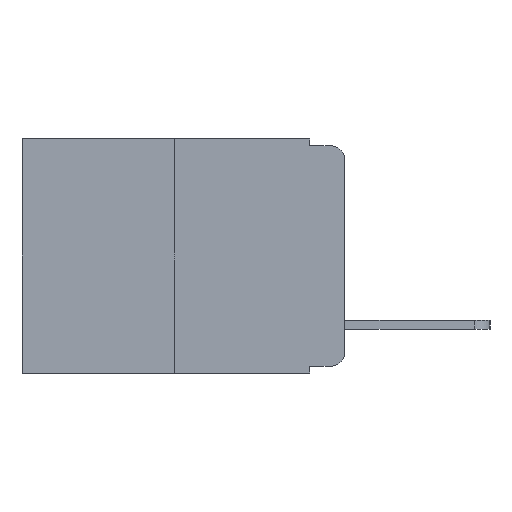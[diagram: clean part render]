
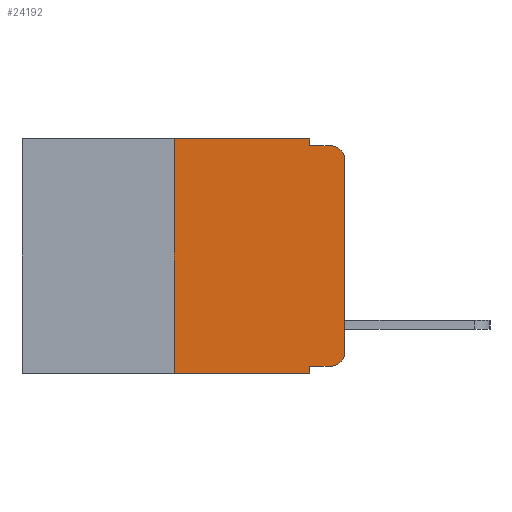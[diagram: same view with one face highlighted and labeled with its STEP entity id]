
A CAD part, left-side view. The second image highlights one B-rep face of the part: STEP entity #24192.
In plain terms, the highlighted planar face has unit normal (-1, 0, 0).
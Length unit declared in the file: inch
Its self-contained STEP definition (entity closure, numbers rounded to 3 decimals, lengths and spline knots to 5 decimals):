
#209 = LINE ( 'NONE', #8318, #15706 ) ;
#849 = DIRECTION ( 'NONE',  ( 0., 0., 1. ) ) ;
#969 = CARTESIAN_POINT ( 'NONE',  ( 0., 0.25, 0. ) ) ;
#1707 = DIRECTION ( 'NONE',  ( 0., -1., 0. ) ) ;
#1868 = AXIS2_PLACEMENT_3D ( 'NONE', #21133, #4867, #19014 ) ;
#2008 = DIRECTION ( 'NONE',  ( 0., 0., -1. ) ) ;
#2235 = ORIENTED_EDGE ( 'NONE', *, *, #18939, .F. ) ;
#2305 = CARTESIAN_POINT ( 'NONE',  ( 0., 0., 0. ) ) ;
#2666 = DIRECTION ( 'NONE',  ( 0., 0., -1. ) ) ;
#2815 = ORIENTED_EDGE ( 'NONE', *, *, #15370, .F. ) ;
#3077 = CIRCLE ( 'NONE', #8180, 0.02 ) ;
#3604 = CIRCLE ( 'NONE', #1868, 0.02 ) ;
#3899 = VERTEX_POINT ( 'NONE', #12358 ) ;
#4414 = VECTOR ( 'NONE', #849, 39.37008 ) ;
#4416 = VECTOR ( 'NONE', #1707, 39.37008 ) ;
#4658 = VERTEX_POINT ( 'NONE', #16699 ) ;
#4867 = DIRECTION ( 'NONE',  ( -1., 0., 0. ) ) ;
#5073 = LINE ( 'NONE', #23183, #23381 ) ;
#5342 = AXIS2_PLACEMENT_3D ( 'NONE', #11040, #7188, #2666 ) ;
#5611 = CARTESIAN_POINT ( 'NONE',  ( 0., 0.051, -0.01 ) ) ;
#5805 = VECTOR ( 'NONE', #12586, 39.37008 ) ;
#5867 = LINE ( 'NONE', #5611, #13993 ) ;
#6166 = EDGE_CURVE ( 'NONE', #4658, #15776, #19712, .T. ) ;
#7188 = DIRECTION ( 'NONE',  ( 1., 0., 0. ) ) ;
#8180 = AXIS2_PLACEMENT_3D ( 'NONE', #20057, #10436, #16259 ) ;
#8318 = CARTESIAN_POINT ( 'NONE',  ( 0., 0.051, 0. ) ) ;
#8396 = EDGE_CURVE ( 'NONE', #3899, #24675, #8898, .T. ) ;
#8898 = LINE ( 'NONE', #20903, #5805 ) ;
#9568 = ORIENTED_EDGE ( 'NONE', *, *, #11268, .T. ) ;
#9883 = VERTEX_POINT ( 'NONE', #20349 ) ;
#10436 = DIRECTION ( 'NONE',  ( -1., 0., 0. ) ) ;
#10524 = EDGE_CURVE ( 'NONE', #22747, #22322, #24782, .T. ) ;
#11040 = CARTESIAN_POINT ( 'NONE',  ( 0., 0.473, 0. ) ) ;
#11268 = EDGE_CURVE ( 'NONE', #15776, #22747, #3604, .T. ) ;
#11978 = DIRECTION ( 'NONE',  ( 0., -1., 0. ) ) ;
#12083 = VERTEX_POINT ( 'NONE', #20386 ) ;
#12358 = CARTESIAN_POINT ( 'NONE',  ( 0., 0.25, 0. ) ) ;
#12586 = DIRECTION ( 'NONE',  ( 0., -1., 0. ) ) ;
#12870 = ORIENTED_EDGE ( 'NONE', *, *, #17074, .T. ) ;
#12884 = EDGE_CURVE ( 'NONE', #22124, #9883, #5867, .T. ) ;
#13495 = CARTESIAN_POINT ( 'NONE',  ( 0., 0.051, -0.343 ) ) ;
#13993 = VECTOR ( 'NONE', #11978, 39.37008 ) ;
#14520 = DIRECTION ( 'NONE',  ( 0., 0., 1. ) ) ;
#14820 = CARTESIAN_POINT ( 'NONE',  ( 0., 0., -0.03 ) ) ;
#15142 = FACE_OUTER_BOUND ( 'NONE', #18280, .T. ) ;
#15259 = VERTEX_POINT ( 'NONE', #13495 ) ;
#15370 = EDGE_CURVE ( 'NONE', #4658, #15259, #209, .T. ) ;
#15493 = ORIENTED_EDGE ( 'NONE', *, *, #10524, .T. ) ;
#15706 = VECTOR ( 'NONE', #24144, 39.37008 ) ;
#15776 = VERTEX_POINT ( 'NONE', #17104 ) ;
#16259 = DIRECTION ( 'NONE',  ( 0., 0., -1. ) ) ;
#16698 = VECTOR ( 'NONE', #14520, 39.37008 ) ;
#16699 = CARTESIAN_POINT ( 'NONE',  ( 0., 0.051, -0.333 ) ) ;
#16884 = CARTESIAN_POINT ( 'NONE',  ( 0., 0., -0.313 ) ) ;
#17074 = EDGE_CURVE ( 'NONE', #22322, #9883, #3077, .T. ) ;
#17104 = CARTESIAN_POINT ( 'NONE',  ( 0., 0.02, -0.333 ) ) ;
#17874 = EDGE_CURVE ( 'NONE', #12083, #15259, #5073, .T. ) ;
#17895 = VECTOR ( 'NONE', #2008, 39.37008 ) ;
#18188 = ORIENTED_EDGE ( 'NONE', *, *, #12884, .F. ) ;
#18280 = EDGE_LOOP ( 'NONE', ( #15493, #12870, #18188, #25420, #26089, #2235, #22436, #2815, #22358, #9568 ) ) ;
#18625 = CARTESIAN_POINT ( 'NONE',  ( 0., 0.051, -0.01 ) ) ;
#18939 = EDGE_CURVE ( 'NONE', #12083, #3899, #22676, .T. ) ;
#19014 = DIRECTION ( 'NONE',  ( 0., 0., -1. ) ) ;
#19222 = EDGE_CURVE ( 'NONE', #24675, #22124, #24228, .T. ) ;
#19712 = LINE ( 'NONE', #21707, #4416 ) ;
#20057 = CARTESIAN_POINT ( 'NONE',  ( 0., 0.02, -0.03 ) ) ;
#20133 = CARTESIAN_POINT ( 'NONE',  ( 0., 0.051, 0. ) ) ;
#20349 = CARTESIAN_POINT ( 'NONE',  ( 0., 0.02, -0.01 ) ) ;
#20386 = CARTESIAN_POINT ( 'NONE',  ( 0., 0.25, -0.343 ) ) ;
#20903 = CARTESIAN_POINT ( 'NONE',  ( 0., 0.473, 0. ) ) ;
#21133 = CARTESIAN_POINT ( 'NONE',  ( 0., 0.02, -0.313 ) ) ;
#21213 = DIRECTION ( 'NONE',  ( 0., -1., 0. ) ) ;
#21707 = CARTESIAN_POINT ( 'NONE',  ( 0., 0.051, -0.333 ) ) ;
#22124 = VERTEX_POINT ( 'NONE', #18625 ) ;
#22322 = VERTEX_POINT ( 'NONE', #14820 ) ;
#22358 = ORIENTED_EDGE ( 'NONE', *, *, #6166, .T. ) ;
#22436 = ORIENTED_EDGE ( 'NONE', *, *, #17874, .T. ) ;
#22676 = LINE ( 'NONE', #969, #4414 ) ;
#22747 = VERTEX_POINT ( 'NONE', #16884 ) ;
#23183 = CARTESIAN_POINT ( 'NONE',  ( 0., 0.473, -0.343 ) ) ;
#23298 = PLANE ( 'NONE',  #5342 ) ;
#23381 = VECTOR ( 'NONE', #21213, 39.37008 ) ;
#24144 = DIRECTION ( 'NONE',  ( 0., 0., -1. ) ) ;
#24192 = ADVANCED_FACE ( 'NONE', ( #15142 ), #23298, .F. ) ;
#24228 = LINE ( 'NONE', #20133, #17895 ) ;
#24675 = VERTEX_POINT ( 'NONE', #24721 ) ;
#24721 = CARTESIAN_POINT ( 'NONE',  ( 0., 0.051, 0. ) ) ;
#24782 = LINE ( 'NONE', #2305, #16698 ) ;
#25420 = ORIENTED_EDGE ( 'NONE', *, *, #19222, .F. ) ;
#26089 = ORIENTED_EDGE ( 'NONE', *, *, #8396, .F. ) ;
